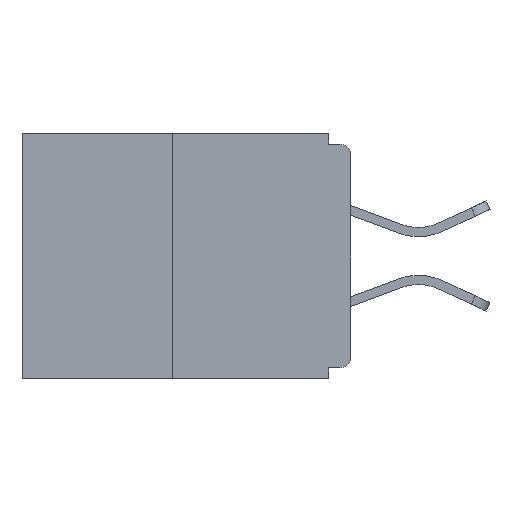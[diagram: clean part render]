
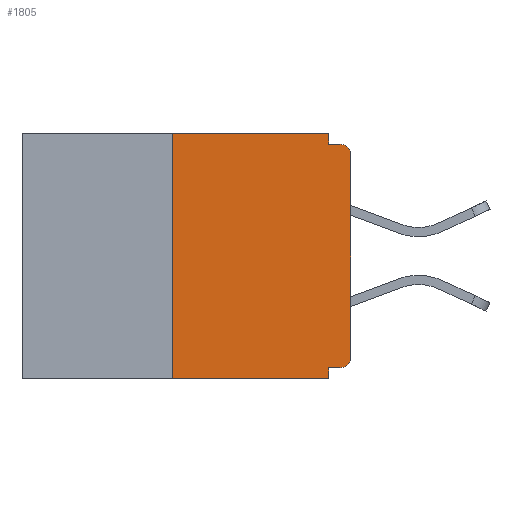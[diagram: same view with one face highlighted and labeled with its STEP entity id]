
A CAD part, left-side view. The second image highlights one B-rep face of the part: STEP entity #1805.
In plain terms, the highlighted planar face has unit normal (-1, 0, 0).
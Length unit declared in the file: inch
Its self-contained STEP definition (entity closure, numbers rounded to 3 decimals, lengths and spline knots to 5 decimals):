
#2 = FACE_OUTER_BOUND ( 'NONE', #18512, .T. ) ;
#257 = CARTESIAN_POINT ( 'NONE',  ( 0., 0.46, -0.343 ) ) ;
#301 = ORIENTED_EDGE ( 'NONE', *, *, #18664, .F. ) ;
#395 = VECTOR ( 'NONE', #2232, 39.37008 ) ;
#473 = DIRECTION ( 'NONE',  ( -1., 0., 0. ) ) ;
#1151 = ORIENTED_EDGE ( 'NONE', *, *, #10009, .F. ) ;
#1250 = CARTESIAN_POINT ( 'NONE',  ( 0., 0.25, 0. ) ) ;
#1375 = VERTEX_POINT ( 'NONE', #20687 ) ;
#1805 = ADVANCED_FACE ( 'NONE', ( #2 ), #15785, .F. ) ;
#1876 = LINE ( 'NONE', #9356, #13988 ) ;
#2012 = ORIENTED_EDGE ( 'NONE', *, *, #15835, .F. ) ;
#2131 = ORIENTED_EDGE ( 'NONE', *, *, #8431, .T. ) ;
#2232 = DIRECTION ( 'NONE',  ( 0., -1., 0. ) ) ;
#2276 = VECTOR ( 'NONE', #15410, 39.37008 ) ;
#2321 = DIRECTION ( 'NONE',  ( 0., 0., -1. ) ) ;
#2331 = LINE ( 'NONE', #7469, #8364 ) ;
#2967 = AXIS2_PLACEMENT_3D ( 'NONE', #10691, #473, #2321 ) ;
#3164 = ORIENTED_EDGE ( 'NONE', *, *, #20959, .T. ) ;
#3228 = CIRCLE ( 'NONE', #2967, 0.015 ) ;
#3618 = VECTOR ( 'NONE', #6545, 39.37008 ) ;
#4117 = CARTESIAN_POINT ( 'NONE',  ( 0., 0.46, 0. ) ) ;
#4526 = LINE ( 'NONE', #1250, #16185 ) ;
#5607 = DIRECTION ( 'NONE',  ( 1., 0., 0. ) ) ;
#5636 = VERTEX_POINT ( 'NONE', #17616 ) ;
#5681 = DIRECTION ( 'NONE',  ( 0., 0., -1. ) ) ;
#5736 = VERTEX_POINT ( 'NONE', #21287 ) ;
#6260 = EDGE_CURVE ( 'NONE', #9595, #18893, #3228, .T. ) ;
#6545 = DIRECTION ( 'NONE',  ( 0., 0., 1. ) ) ;
#7092 = DIRECTION ( 'NONE',  ( 0., -1., 0. ) ) ;
#7181 = ORIENTED_EDGE ( 'NONE', *, *, #14240, .F. ) ;
#7438 = EDGE_CURVE ( 'NONE', #5736, #1375, #14488, .T. ) ;
#7469 = CARTESIAN_POINT ( 'NONE',  ( 0., 0.031, 0. ) ) ;
#8093 = DIRECTION ( 'NONE',  ( -1., 0., 0. ) ) ;
#8364 = VECTOR ( 'NONE', #15840, 39.37008 ) ;
#8431 = EDGE_CURVE ( 'NONE', #10192, #5636, #21107, .T. ) ;
#8460 = EDGE_CURVE ( 'NONE', #16724, #12728, #2331, .T. ) ;
#8540 = CARTESIAN_POINT ( 'NONE',  ( 0., 0.015, -0.015 ) ) ;
#9356 = CARTESIAN_POINT ( 'NONE',  ( 0., 0., -0.015 ) ) ;
#9496 = ORIENTED_EDGE ( 'NONE', *, *, #7438, .T. ) ;
#9595 = VERTEX_POINT ( 'NONE', #15834 ) ;
#9890 = VERTEX_POINT ( 'NONE', #10173 ) ;
#10009 = EDGE_CURVE ( 'NONE', #13418, #16724, #11982, .T. ) ;
#10173 = CARTESIAN_POINT ( 'NONE',  ( 0., 0.031, -0.328 ) ) ;
#10192 = VERTEX_POINT ( 'NONE', #12886 ) ;
#10671 = ORIENTED_EDGE ( 'NONE', *, *, #17106, .F. ) ;
#10691 = CARTESIAN_POINT ( 'NONE',  ( 0., 0.015, -0.03 ) ) ;
#10931 = LINE ( 'NONE', #18751, #2276 ) ;
#11982 = LINE ( 'NONE', #14086, #395 ) ;
#12728 = VERTEX_POINT ( 'NONE', #14006 ) ;
#12801 = DIRECTION ( 'NONE',  ( 0., 0., 1. ) ) ;
#12886 = CARTESIAN_POINT ( 'NONE',  ( 0., 0.25, -0.343 ) ) ;
#13007 = AXIS2_PLACEMENT_3D ( 'NONE', #16561, #8093, #19662 ) ;
#13418 = VERTEX_POINT ( 'NONE', #21844 ) ;
#13869 = ORIENTED_EDGE ( 'NONE', *, *, #8460, .F. ) ;
#13988 = VECTOR ( 'NONE', #17676, 39.37008 ) ;
#14006 = CARTESIAN_POINT ( 'NONE',  ( 0., 0.031, -0.015 ) ) ;
#14086 = CARTESIAN_POINT ( 'NONE',  ( 0., 0.46, 0. ) ) ;
#14240 = EDGE_CURVE ( 'NONE', #9890, #5636, #10931, .T. ) ;
#14488 = CIRCLE ( 'NONE', #13007, 0.015 ) ;
#14898 = CARTESIAN_POINT ( 'NONE',  ( 0., 0., 0. ) ) ;
#15146 = CARTESIAN_POINT ( 'NONE',  ( 0., 0.031, 0. ) ) ;
#15410 = DIRECTION ( 'NONE',  ( 0., 0., -1. ) ) ;
#15785 = PLANE ( 'NONE',  #19898 ) ;
#15834 = CARTESIAN_POINT ( 'NONE',  ( 0., 0., -0.03 ) ) ;
#15835 = EDGE_CURVE ( 'NONE', #10192, #13418, #4526, .T. ) ;
#15840 = DIRECTION ( 'NONE',  ( 0., 0., -1. ) ) ;
#16185 = VECTOR ( 'NONE', #12801, 39.37008 ) ;
#16561 = CARTESIAN_POINT ( 'NONE',  ( 0., 0.015, -0.313 ) ) ;
#16724 = VERTEX_POINT ( 'NONE', #15146 ) ;
#17106 = EDGE_CURVE ( 'NONE', #12728, #18893, #1876, .T. ) ;
#17616 = CARTESIAN_POINT ( 'NONE',  ( 0., 0.031, -0.343 ) ) ;
#17676 = DIRECTION ( 'NONE',  ( 0., -1., 0. ) ) ;
#18512 = EDGE_LOOP ( 'NONE', ( #1151, #2012, #2131, #7181, #301, #9496, #3164, #20706, #10671, #13869 ) ) ;
#18664 = EDGE_CURVE ( 'NONE', #5736, #9890, #19500, .T. ) ;
#18751 = CARTESIAN_POINT ( 'NONE',  ( 0., 0.031, -0.343 ) ) ;
#18893 = VERTEX_POINT ( 'NONE', #8540 ) ;
#19500 = LINE ( 'NONE', #19652, #21096 ) ;
#19652 = CARTESIAN_POINT ( 'NONE',  ( 0., 0., -0.328 ) ) ;
#19662 = DIRECTION ( 'NONE',  ( 0., 0., -1. ) ) ;
#19735 = LINE ( 'NONE', #14898, #3618 ) ;
#19898 = AXIS2_PLACEMENT_3D ( 'NONE', #4117, #5607, #5681 ) ;
#20687 = CARTESIAN_POINT ( 'NONE',  ( 0., 0., -0.313 ) ) ;
#20706 = ORIENTED_EDGE ( 'NONE', *, *, #6260, .T. ) ;
#20833 = VECTOR ( 'NONE', #7092, 39.37008 ) ;
#20959 = EDGE_CURVE ( 'NONE', #1375, #9595, #19735, .T. ) ;
#21096 = VECTOR ( 'NONE', #21421, 39.37008 ) ;
#21107 = LINE ( 'NONE', #257, #20833 ) ;
#21287 = CARTESIAN_POINT ( 'NONE',  ( 0., 0.015, -0.328 ) ) ;
#21421 = DIRECTION ( 'NONE',  ( 0., 1., 0. ) ) ;
#21844 = CARTESIAN_POINT ( 'NONE',  ( 0., 0.25, 0. ) ) ;
